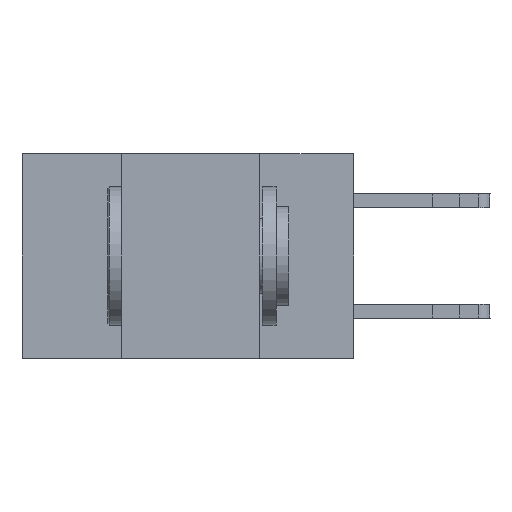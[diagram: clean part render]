
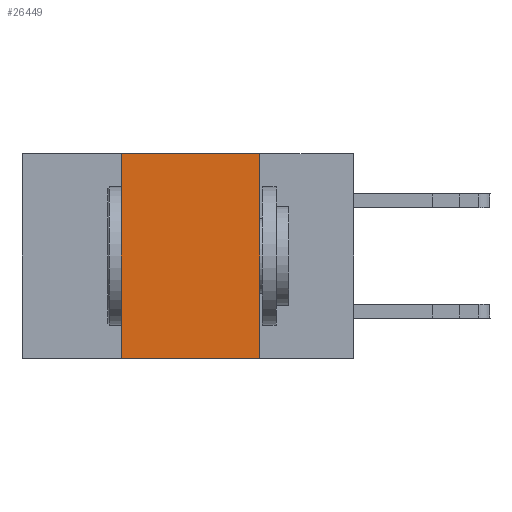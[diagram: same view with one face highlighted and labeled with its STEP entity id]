
A CAD part, left-side view. The second image highlights one B-rep face of the part: STEP entity #26449.
In plain terms, the highlighted planar face has unit normal (-1, 0, 0).
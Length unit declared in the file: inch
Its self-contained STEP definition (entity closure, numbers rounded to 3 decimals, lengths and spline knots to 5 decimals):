
#713 = ORIENTED_EDGE ( 'NONE', *, *, #2355, .F. ) ;
#1446 = LINE ( 'NONE', #8502, #26971 ) ;
#1848 = EDGE_CURVE ( 'NONE', #17139, #16120, #16051, .T. ) ;
#2355 = EDGE_CURVE ( 'NONE', #17139, #27118, #9272, .T. ) ;
#3162 = EDGE_LOOP ( 'NONE', ( #27157, #21464, #713, #10055 ) ) ;
#3482 = LINE ( 'NONE', #16562, #29019 ) ;
#5899 = CARTESIAN_POINT ( 'NONE',  ( 0., 0.6, -0.37 ) ) ;
#5929 = DIRECTION ( 'NONE',  ( 0., 0., -1. ) ) ;
#8283 = FACE_OUTER_BOUND ( 'NONE', #3162, .T. ) ;
#8317 = AXIS2_PLACEMENT_3D ( 'NONE', #23116, #13488, #5929 ) ;
#8321 = CARTESIAN_POINT ( 'NONE',  ( 0., 0.42, 0. ) ) ;
#8502 = CARTESIAN_POINT ( 'NONE',  ( 0., 0.6, 0. ) ) ;
#9272 = LINE ( 'NONE', #8321, #21312 ) ;
#10055 = ORIENTED_EDGE ( 'NONE', *, *, #1848, .T. ) ;
#10901 = DIRECTION ( 'NONE',  ( 0., -1., 0. ) ) ;
#13488 = DIRECTION ( 'NONE',  ( 1., 0., 0. ) ) ;
#16051 = LINE ( 'NONE', #5899, #20562 ) ;
#16120 = VERTEX_POINT ( 'NONE', #22733 ) ;
#16562 = CARTESIAN_POINT ( 'NONE',  ( 0., 0.17, 0. ) ) ;
#16656 = CARTESIAN_POINT ( 'NONE',  ( 0., 0.17, 0. ) ) ;
#17139 = VERTEX_POINT ( 'NONE', #17516 ) ;
#17516 = CARTESIAN_POINT ( 'NONE',  ( 0., 0.42, -0.37 ) ) ;
#17988 = DIRECTION ( 'NONE',  ( 0., -1., 0. ) ) ;
#19402 = DIRECTION ( 'NONE',  ( 0., 0., -1. ) ) ;
#20562 = VECTOR ( 'NONE', #17988, 39.37008 ) ;
#21312 = VECTOR ( 'NONE', #24812, 39.37008 ) ;
#21347 = VERTEX_POINT ( 'NONE', #16656 ) ;
#21464 = ORIENTED_EDGE ( 'NONE', *, *, #22364, .F. ) ;
#22364 = EDGE_CURVE ( 'NONE', #27118, #21347, #1446, .T. ) ;
#22733 = CARTESIAN_POINT ( 'NONE',  ( 0., 0.17, -0.37 ) ) ;
#23116 = CARTESIAN_POINT ( 'NONE',  ( 0., 0.6, 0. ) ) ;
#23661 = CARTESIAN_POINT ( 'NONE',  ( 0., 0.42, 0. ) ) ;
#24812 = DIRECTION ( 'NONE',  ( 0., 0., 1. ) ) ;
#26449 = ADVANCED_FACE ( 'NONE', ( #8283 ), #27541, .F. ) ;
#26971 = VECTOR ( 'NONE', #10901, 39.37008 ) ;
#27118 = VERTEX_POINT ( 'NONE', #23661 ) ;
#27157 = ORIENTED_EDGE ( 'NONE', *, *, #30582, .F. ) ;
#27541 = PLANE ( 'NONE',  #8317 ) ;
#29019 = VECTOR ( 'NONE', #19402, 39.37008 ) ;
#30582 = EDGE_CURVE ( 'NONE', #21347, #16120, #3482, .T. ) ;
